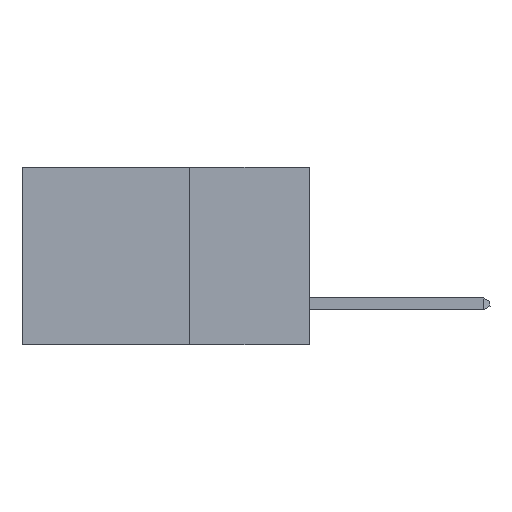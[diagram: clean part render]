
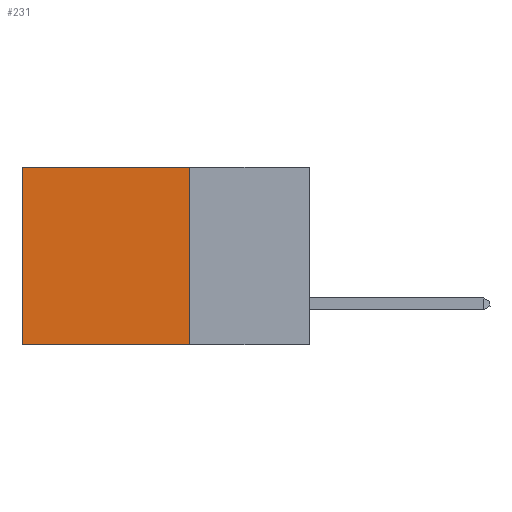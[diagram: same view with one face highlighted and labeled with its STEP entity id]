
A CAD part, left-side view. The second image highlights one B-rep face of the part: STEP entity #231.
In plain terms, the highlighted planar face has unit normal (-1, 0, 0).
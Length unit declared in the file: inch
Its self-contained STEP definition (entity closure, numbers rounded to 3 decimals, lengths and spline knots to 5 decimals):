
#37 = LINE ( 'NONE', #13711, #12301 ) ;
#146 = VECTOR ( 'NONE', #14531, 39.37008 ) ;
#231 = ADVANCED_FACE ( 'NONE', ( #10703 ), #11465, .F. ) ;
#305 = VECTOR ( 'NONE', #4148, 39.37008 ) ;
#506 = EDGE_CURVE ( 'NONE', #11846, #12925, #12233, .T. ) ;
#835 = CARTESIAN_POINT ( 'NONE',  ( 0.2875, 0.6, 0. ) ) ;
#1673 = DIRECTION ( 'NONE',  ( 0., 0., -1. ) ) ;
#1760 = AXIS2_PLACEMENT_3D ( 'NONE', #12836, #13953, #1673 ) ;
#2223 = EDGE_LOOP ( 'NONE', ( #12590, #3595, #9481, #9043 ) ) ;
#3595 = ORIENTED_EDGE ( 'NONE', *, *, #3972, .F. ) ;
#3972 = EDGE_CURVE ( 'NONE', #5037, #12925, #37, .T. ) ;
#4116 = DIRECTION ( 'NONE',  ( 0., 1., 0. ) ) ;
#4148 = DIRECTION ( 'NONE',  ( 0., 1., 0. ) ) ;
#4292 = VERTEX_POINT ( 'NONE', #5354 ) ;
#5020 = EDGE_CURVE ( 'NONE', #4292, #11846, #5573, .T. ) ;
#5037 = VERTEX_POINT ( 'NONE', #6792 ) ;
#5354 = CARTESIAN_POINT ( 'NONE',  ( 0.2875, 0.25, 0. ) ) ;
#5358 = LINE ( 'NONE', #11684, #6157 ) ;
#5573 = LINE ( 'NONE', #7942, #305 ) ;
#6157 = VECTOR ( 'NONE', #10135, 39.37008 ) ;
#6792 = CARTESIAN_POINT ( 'NONE',  ( 0.2875, 0.25, -0.37 ) ) ;
#7942 = CARTESIAN_POINT ( 'NONE',  ( 0.2875, 0.25, 0. ) ) ;
#7948 = CARTESIAN_POINT ( 'NONE',  ( 0.2875, 0.6, -0.37 ) ) ;
#9043 = ORIENTED_EDGE ( 'NONE', *, *, #5020, .T. ) ;
#9481 = ORIENTED_EDGE ( 'NONE', *, *, #10987, .F. ) ;
#10135 = DIRECTION ( 'NONE',  ( 0., 0., -1. ) ) ;
#10703 = FACE_OUTER_BOUND ( 'NONE', #2223, .T. ) ;
#10987 = EDGE_CURVE ( 'NONE', #4292, #5037, #5358, .T. ) ;
#11364 = CARTESIAN_POINT ( 'NONE',  ( 0.2875, 0.6, 0. ) ) ;
#11465 = PLANE ( 'NONE',  #1760 ) ;
#11684 = CARTESIAN_POINT ( 'NONE',  ( 0.2875, 0.25, 0. ) ) ;
#11846 = VERTEX_POINT ( 'NONE', #11364 ) ;
#12233 = LINE ( 'NONE', #835, #146 ) ;
#12301 = VECTOR ( 'NONE', #4116, 39.37008 ) ;
#12590 = ORIENTED_EDGE ( 'NONE', *, *, #506, .T. ) ;
#12836 = CARTESIAN_POINT ( 'NONE',  ( 0.2875, 0.25, 0. ) ) ;
#12925 = VERTEX_POINT ( 'NONE', #7948 ) ;
#13711 = CARTESIAN_POINT ( 'NONE',  ( 0.2875, 0.25, -0.37 ) ) ;
#13953 = DIRECTION ( 'NONE',  ( 1., 0., 0. ) ) ;
#14531 = DIRECTION ( 'NONE',  ( 0., 0., -1. ) ) ;
